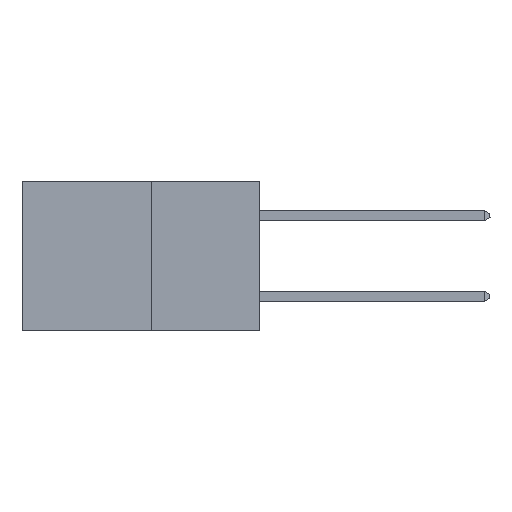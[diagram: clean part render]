
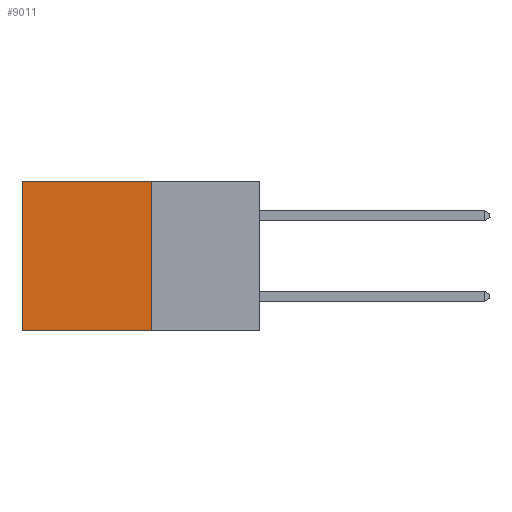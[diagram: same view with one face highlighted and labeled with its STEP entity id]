
A CAD part, left-side view. The second image highlights one B-rep face of the part: STEP entity #9011.
In plain terms, the highlighted planar face has unit normal (-1, 0, 0).
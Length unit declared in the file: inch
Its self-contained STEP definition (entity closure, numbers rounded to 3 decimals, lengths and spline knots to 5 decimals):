
#62 = VECTOR ( 'NONE', #7813, 39.37008 ) ;
#86 = VERTEX_POINT ( 'NONE', #7526 ) ;
#545 = LINE ( 'NONE', #16803, #62 ) ;
#1090 = EDGE_LOOP ( 'NONE', ( #15721, #12161, #1641, #7731 ) ) ;
#1641 = ORIENTED_EDGE ( 'NONE', *, *, #9698, .F. ) ;
#2405 = DIRECTION ( 'NONE',  ( 0., 1., 0. ) ) ;
#2852 = VECTOR ( 'NONE', #2405, 39.37008 ) ;
#4676 = LINE ( 'NONE', #18868, #16211 ) ;
#5491 = VERTEX_POINT ( 'NONE', #17585 ) ;
#6738 = VECTOR ( 'NONE', #13420, 39.37008 ) ;
#6924 = EDGE_CURVE ( 'NONE', #13130, #18218, #10803, .T. ) ;
#7526 = CARTESIAN_POINT ( 'NONE',  ( 0.277, 0.59, -0.37 ) ) ;
#7731 = ORIENTED_EDGE ( 'NONE', *, *, #6924, .T. ) ;
#7745 = CARTESIAN_POINT ( 'NONE',  ( 0.277, 0.59, 0. ) ) ;
#7813 = DIRECTION ( 'NONE',  ( 0., 0., -1. ) ) ;
#8466 = PLANE ( 'NONE',  #12785 ) ;
#9011 = ADVANCED_FACE ( 'NONE', ( #11701 ), #8466, .F. ) ;
#9598 = CARTESIAN_POINT ( 'NONE',  ( 0.277, 0.27, 0. ) ) ;
#9698 = EDGE_CURVE ( 'NONE', #13130, #5491, #17746, .T. ) ;
#10118 = DIRECTION ( 'NONE',  ( 0., 0., -1. ) ) ;
#10803 = LINE ( 'NONE', #14276, #2852 ) ;
#11230 = EDGE_CURVE ( 'NONE', #5491, #86, #4676, .T. ) ;
#11701 = FACE_OUTER_BOUND ( 'NONE', #1090, .T. ) ;
#12161 = ORIENTED_EDGE ( 'NONE', *, *, #11230, .F. ) ;
#12463 = DIRECTION ( 'NONE',  ( 1., 0., 0. ) ) ;
#12484 = CARTESIAN_POINT ( 'NONE',  ( 0.277, 0.27, -0.37 ) ) ;
#12785 = AXIS2_PLACEMENT_3D ( 'NONE', #12484, #12463, #10118 ) ;
#13130 = VERTEX_POINT ( 'NONE', #9598 ) ;
#13420 = DIRECTION ( 'NONE',  ( 0., 0., -1. ) ) ;
#14276 = CARTESIAN_POINT ( 'NONE',  ( 0.277, 0.27, 0. ) ) ;
#15721 = ORIENTED_EDGE ( 'NONE', *, *, #16082, .T. ) ;
#16082 = EDGE_CURVE ( 'NONE', #18218, #86, #545, .T. ) ;
#16211 = VECTOR ( 'NONE', #18500, 39.37008 ) ;
#16803 = CARTESIAN_POINT ( 'NONE',  ( 0.277, 0.59, -0.37 ) ) ;
#17585 = CARTESIAN_POINT ( 'NONE',  ( 0.277, 0.27, -0.37 ) ) ;
#17746 = LINE ( 'NONE', #18293, #6738 ) ;
#18218 = VERTEX_POINT ( 'NONE', #7745 ) ;
#18293 = CARTESIAN_POINT ( 'NONE',  ( 0.277, 0.27, -0.37 ) ) ;
#18500 = DIRECTION ( 'NONE',  ( 0., 1., 0. ) ) ;
#18868 = CARTESIAN_POINT ( 'NONE',  ( 0.277, 0.27, -0.37 ) ) ;
